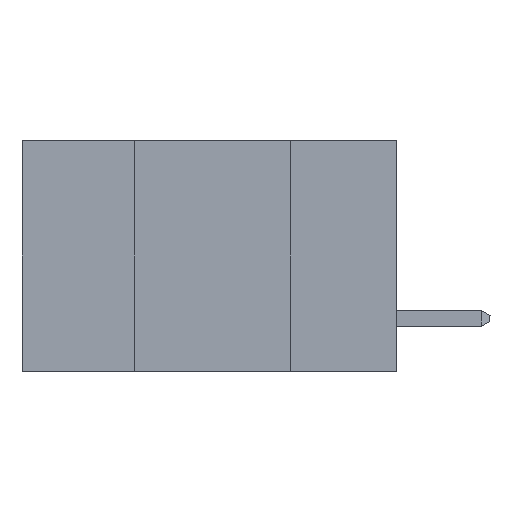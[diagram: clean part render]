
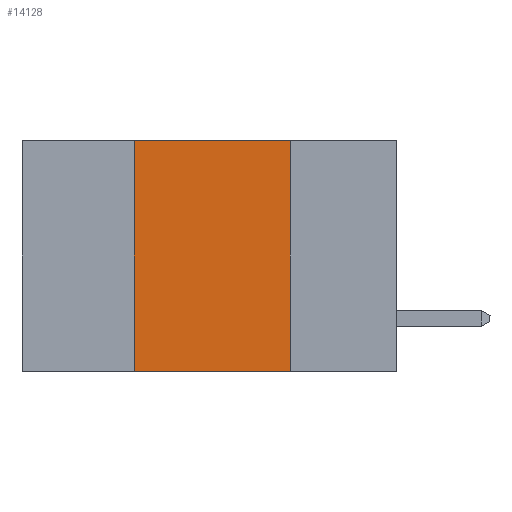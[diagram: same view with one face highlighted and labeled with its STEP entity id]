
A CAD part, left-side view. The second image highlights one B-rep face of the part: STEP entity #14128.
In plain terms, the highlighted planar face has unit normal (-1, 0, 0).
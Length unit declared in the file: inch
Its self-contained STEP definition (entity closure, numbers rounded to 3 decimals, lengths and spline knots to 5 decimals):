
#1187 = DIRECTION ( 'NONE',  ( 0., -1., 0. ) ) ;
#1206 = LINE ( 'NONE', #21752, #5757 ) ;
#1336 = DIRECTION ( 'NONE',  ( 1., 0., 0. ) ) ;
#1586 = LINE ( 'NONE', #9423, #21131 ) ;
#3528 = CARTESIAN_POINT ( 'NONE',  ( 0., 0.6, 0. ) ) ;
#4214 = AXIS2_PLACEMENT_3D ( 'NONE', #3528, #1336, #22222 ) ;
#4872 = EDGE_CURVE ( 'NONE', #23945, #19620, #8792, .T. ) ;
#5757 = VECTOR ( 'NONE', #11394, 39.37008 ) ;
#6484 = CARTESIAN_POINT ( 'NONE',  ( 0., 0.17, 0. ) ) ;
#8196 = ORIENTED_EDGE ( 'NONE', *, *, #4872, .T. ) ;
#8761 = VECTOR ( 'NONE', #12873, 39.37008 ) ;
#8792 = LINE ( 'NONE', #24872, #25853 ) ;
#9423 = CARTESIAN_POINT ( 'NONE',  ( 0., 0.6, 0. ) ) ;
#9778 = CARTESIAN_POINT ( 'NONE',  ( 0., 0.42, 0. ) ) ;
#9960 = CARTESIAN_POINT ( 'NONE',  ( 0., 0.17, 0. ) ) ;
#11394 = DIRECTION ( 'NONE',  ( 0., 0., 1. ) ) ;
#12084 = CARTESIAN_POINT ( 'NONE',  ( 0., 0.17, -0.37 ) ) ;
#12406 = DIRECTION ( 'NONE',  ( 0., -1., 0. ) ) ;
#12873 = DIRECTION ( 'NONE',  ( 0., 0., -1. ) ) ;
#12885 = EDGE_LOOP ( 'NONE', ( #26863, #22846, #19299, #8196 ) ) ;
#14128 = ADVANCED_FACE ( 'NONE', ( #18040 ), #22132, .F. ) ;
#14417 = LINE ( 'NONE', #6484, #8761 ) ;
#17043 = VERTEX_POINT ( 'NONE', #9778 ) ;
#18040 = FACE_OUTER_BOUND ( 'NONE', #12885, .T. ) ;
#19299 = ORIENTED_EDGE ( 'NONE', *, *, #25337, .F. ) ;
#19620 = VERTEX_POINT ( 'NONE', #12084 ) ;
#20812 = EDGE_CURVE ( 'NONE', #25473, #19620, #14417, .T. ) ;
#21131 = VECTOR ( 'NONE', #1187, 39.37008 ) ;
#21752 = CARTESIAN_POINT ( 'NONE',  ( 0., 0.42, 0. ) ) ;
#22132 = PLANE ( 'NONE',  #4214 ) ;
#22222 = DIRECTION ( 'NONE',  ( 0., 0., -1. ) ) ;
#22240 = EDGE_CURVE ( 'NONE', #17043, #25473, #1586, .T. ) ;
#22846 = ORIENTED_EDGE ( 'NONE', *, *, #22240, .F. ) ;
#23654 = CARTESIAN_POINT ( 'NONE',  ( 0., 0.42, -0.37 ) ) ;
#23945 = VERTEX_POINT ( 'NONE', #23654 ) ;
#24872 = CARTESIAN_POINT ( 'NONE',  ( 0., 0.6, -0.37 ) ) ;
#25337 = EDGE_CURVE ( 'NONE', #23945, #17043, #1206, .T. ) ;
#25473 = VERTEX_POINT ( 'NONE', #9960 ) ;
#25853 = VECTOR ( 'NONE', #12406, 39.37008 ) ;
#26863 = ORIENTED_EDGE ( 'NONE', *, *, #20812, .F. ) ;
